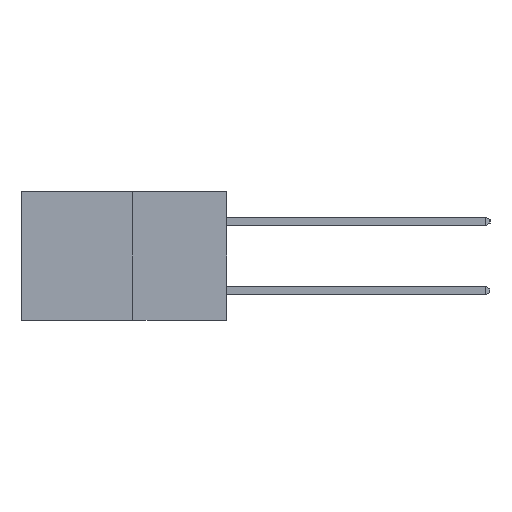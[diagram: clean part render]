
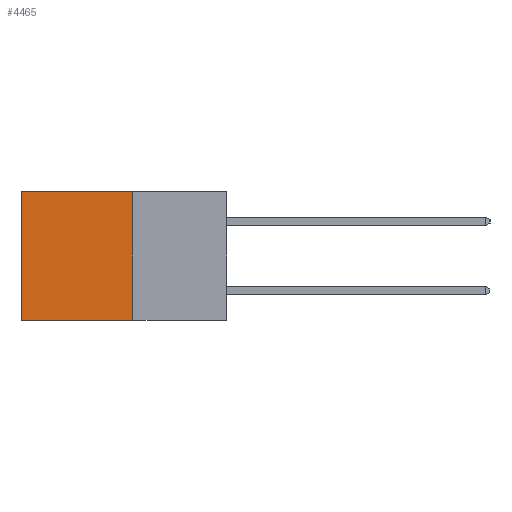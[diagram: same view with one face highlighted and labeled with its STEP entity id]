
A CAD part, left-side view. The second image highlights one B-rep face of the part: STEP entity #4465.
In plain terms, the highlighted planar face has unit normal (-1, 0, 0).
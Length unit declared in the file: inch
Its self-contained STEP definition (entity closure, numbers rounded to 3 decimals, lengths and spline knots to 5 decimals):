
#39 = ORIENTED_EDGE ( 'NONE', *, *, #14791, .F. ) ;
#786 = LINE ( 'NONE', #8972, #15543 ) ;
#976 = CARTESIAN_POINT ( 'NONE',  ( 0.277, 0.59, -0.37 ) ) ;
#1060 = VECTOR ( 'NONE', #1313, 39.37008 ) ;
#1225 = VERTEX_POINT ( 'NONE', #17577 ) ;
#1313 = DIRECTION ( 'NONE',  ( 0., 0., -1. ) ) ;
#1598 = FACE_OUTER_BOUND ( 'NONE', #17821, .T. ) ;
#2224 = LINE ( 'NONE', #13338, #10778 ) ;
#3441 = ORIENTED_EDGE ( 'NONE', *, *, #17392, .F. ) ;
#4124 = ORIENTED_EDGE ( 'NONE', *, *, #7506, .T. ) ;
#4250 = VECTOR ( 'NONE', #14446, 39.37008 ) ;
#4465 = ADVANCED_FACE ( 'NONE', ( #1598 ), #8587, .F. ) ;
#4687 = DIRECTION ( 'NONE',  ( 0., 1., 0. ) ) ;
#6283 = CARTESIAN_POINT ( 'NONE',  ( 0.277, 0.59, 0. ) ) ;
#6523 = VERTEX_POINT ( 'NONE', #6283 ) ;
#7506 = EDGE_CURVE ( 'NONE', #6523, #8064, #9200, .T. ) ;
#7801 = CARTESIAN_POINT ( 'NONE',  ( 0.277, 0.27, 0. ) ) ;
#8064 = VERTEX_POINT ( 'NONE', #976 ) ;
#8136 = LINE ( 'NONE', #11606, #4250 ) ;
#8587 = PLANE ( 'NONE',  #16371 ) ;
#8752 = DIRECTION ( 'NONE',  ( 0., 0., -1. ) ) ;
#8972 = CARTESIAN_POINT ( 'NONE',  ( 0.277, 0.27, -0.37 ) ) ;
#9200 = LINE ( 'NONE', #15616, #1060 ) ;
#10365 = DIRECTION ( 'NONE',  ( 1., 0., 0. ) ) ;
#10778 = VECTOR ( 'NONE', #4687, 39.37008 ) ;
#11075 = CARTESIAN_POINT ( 'NONE',  ( 0.277, 0.27, -0.37 ) ) ;
#11557 = ORIENTED_EDGE ( 'NONE', *, *, #14296, .T. ) ;
#11606 = CARTESIAN_POINT ( 'NONE',  ( 0.277, 0.27, -0.37 ) ) ;
#13338 = CARTESIAN_POINT ( 'NONE',  ( 0.277, 0.27, 0. ) ) ;
#13623 = VERTEX_POINT ( 'NONE', #7801 ) ;
#14296 = EDGE_CURVE ( 'NONE', #13623, #6523, #2224, .T. ) ;
#14446 = DIRECTION ( 'NONE',  ( 0., 0., -1. ) ) ;
#14791 = EDGE_CURVE ( 'NONE', #13623, #1225, #8136, .T. ) ;
#15543 = VECTOR ( 'NONE', #16018, 39.37008 ) ;
#15616 = CARTESIAN_POINT ( 'NONE',  ( 0.277, 0.59, -0.37 ) ) ;
#16018 = DIRECTION ( 'NONE',  ( 0., 1., 0. ) ) ;
#16371 = AXIS2_PLACEMENT_3D ( 'NONE', #11075, #10365, #8752 ) ;
#17392 = EDGE_CURVE ( 'NONE', #1225, #8064, #786, .T. ) ;
#17577 = CARTESIAN_POINT ( 'NONE',  ( 0.277, 0.27, -0.37 ) ) ;
#17821 = EDGE_LOOP ( 'NONE', ( #4124, #3441, #39, #11557 ) ) ;
